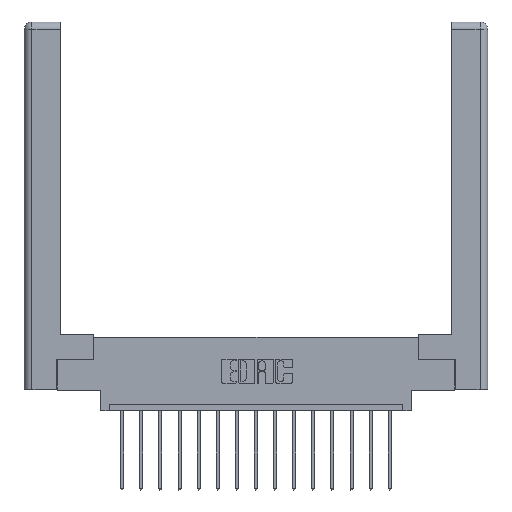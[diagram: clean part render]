
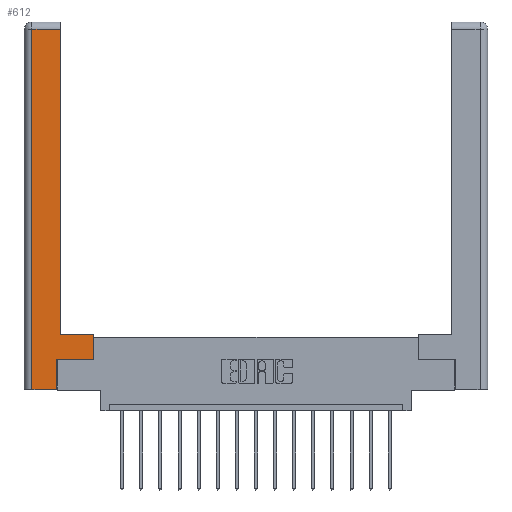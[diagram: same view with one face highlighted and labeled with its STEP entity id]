
A CAD part, top view. The second image highlights one B-rep face of the part: STEP entity #612.
In plain terms, the highlighted planar face has unit normal (0, 0, 1).
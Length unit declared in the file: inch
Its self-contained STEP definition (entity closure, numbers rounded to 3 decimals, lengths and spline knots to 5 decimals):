
#231 = VECTOR ( 'NONE', #6738, 39.37008 ) ;
#248 = CARTESIAN_POINT ( 'NONE',  ( 0.0615, 2.94, 0. ) ) ;
#262 = VECTOR ( 'NONE', #8259, 39.37008 ) ;
#455 = LINE ( 'NONE', #5295, #231 ) ;
#593 = AXIS2_PLACEMENT_3D ( 'NONE', #5013, #2111, #3486 ) ;
#612 = ADVANCED_FACE ( 'NONE', ( #8529 ), #7703, .F. ) ;
#699 = VECTOR ( 'NONE', #1119, 39.37008 ) ;
#715 = CARTESIAN_POINT ( 'NONE',  ( 0.295, 0.45, 0. ) ) ;
#750 = CARTESIAN_POINT ( 'NONE',  ( 0.565, 0.245, 0. ) ) ;
#1115 = ORIENTED_EDGE ( 'NONE', *, *, #2003, .T. ) ;
#1119 = DIRECTION ( 'NONE',  ( 0., 1., 0. ) ) ;
#1220 = EDGE_CURVE ( 'NONE', #11524, #2676, #3639, .T. ) ;
#2003 = EDGE_CURVE ( 'NONE', #2617, #9359, #12914, .T. ) ;
#2111 = DIRECTION ( 'NONE',  ( 0., 0., -1. ) ) ;
#2519 = DIRECTION ( 'NONE',  ( 0., 1., 0. ) ) ;
#2617 = VERTEX_POINT ( 'NONE', #13275 ) ;
#2668 = CARTESIAN_POINT ( 'NONE',  ( 0.565, 0.245, 0. ) ) ;
#2676 = VERTEX_POINT ( 'NONE', #3179 ) ;
#3179 = CARTESIAN_POINT ( 'NONE',  ( 0.265, 0., 0. ) ) ;
#3486 = DIRECTION ( 'NONE',  ( -1., 0., 0. ) ) ;
#3639 = LINE ( 'NONE', #13524, #10410 ) ;
#3986 = EDGE_CURVE ( 'NONE', #10735, #13105, #10806, .T. ) ;
#4422 = ORIENTED_EDGE ( 'NONE', *, *, #3986, .T. ) ;
#5013 = CARTESIAN_POINT ( 'NONE',  ( 0., 0., 0. ) ) ;
#5295 = CARTESIAN_POINT ( 'NONE',  ( 0.0615, 0., 0. ) ) ;
#5396 = ORIENTED_EDGE ( 'NONE', *, *, #7815, .T. ) ;
#5695 = ORIENTED_EDGE ( 'NONE', *, *, #13593, .T. ) ;
#5744 = LINE ( 'NONE', #2668, #262 ) ;
#5765 = ORIENTED_EDGE ( 'NONE', *, *, #1220, .T. ) ;
#6270 = VECTOR ( 'NONE', #7347, 39.37008 ) ;
#6445 = CARTESIAN_POINT ( 'NONE',  ( 0.295, 2.94, 0. ) ) ;
#6547 = EDGE_LOOP ( 'NONE', ( #1115, #6872, #5695, #5765, #7364, #7105, #4422, #5396 ) ) ;
#6738 = DIRECTION ( 'NONE',  ( 0., -1., 0. ) ) ;
#6872 = ORIENTED_EDGE ( 'NONE', *, *, #16805, .T. ) ;
#7064 = CARTESIAN_POINT ( 'NONE',  ( 0.565, 0.45, 0. ) ) ;
#7105 = ORIENTED_EDGE ( 'NONE', *, *, #12953, .T. ) ;
#7244 = VECTOR ( 'NONE', #2519, 39.37008 ) ;
#7347 = DIRECTION ( 'NONE',  ( -1., 0., 0. ) ) ;
#7364 = ORIENTED_EDGE ( 'NONE', *, *, #12517, .T. ) ;
#7703 = PLANE ( 'NONE',  #593 ) ;
#7815 = EDGE_CURVE ( 'NONE', #13105, #2617, #11560, .T. ) ;
#8259 = DIRECTION ( 'NONE',  ( 1., 0., 0. ) ) ;
#8529 = FACE_OUTER_BOUND ( 'NONE', #6547, .T. ) ;
#9359 = VERTEX_POINT ( 'NONE', #6445 ) ;
#9709 = CARTESIAN_POINT ( 'NONE',  ( 0.565, 0.45, 0. ) ) ;
#9745 = DIRECTION ( 'NONE',  ( -1., 0., 0. ) ) ;
#10025 = VECTOR ( 'NONE', #9745, 39.37008 ) ;
#10357 = CARTESIAN_POINT ( 'NONE',  ( 0.0615, 0., 0. ) ) ;
#10410 = VECTOR ( 'NONE', #15086, 39.37008 ) ;
#10695 = VERTEX_POINT ( 'NONE', #16728 ) ;
#10735 = VERTEX_POINT ( 'NONE', #750 ) ;
#10806 = LINE ( 'NONE', #9709, #12285 ) ;
#11269 = LINE ( 'NONE', #16097, #699 ) ;
#11524 = VERTEX_POINT ( 'NONE', #10357 ) ;
#11560 = LINE ( 'NONE', #715, #6270 ) ;
#12233 = VERTEX_POINT ( 'NONE', #12720 ) ;
#12285 = VECTOR ( 'NONE', #12486, 39.37008 ) ;
#12486 = DIRECTION ( 'NONE',  ( 0., 1., 0. ) ) ;
#12517 = EDGE_CURVE ( 'NONE', #2676, #12233, #11269, .T. ) ;
#12720 = CARTESIAN_POINT ( 'NONE',  ( 0.265, 0.245, 0. ) ) ;
#12914 = LINE ( 'NONE', #14315, #7244 ) ;
#12953 = EDGE_CURVE ( 'NONE', #12233, #10735, #5744, .T. ) ;
#13105 = VERTEX_POINT ( 'NONE', #7064 ) ;
#13275 = CARTESIAN_POINT ( 'NONE',  ( 0.295, 0.45, 0. ) ) ;
#13524 = CARTESIAN_POINT ( 'NONE',  ( 0.265, 0., 0. ) ) ;
#13593 = EDGE_CURVE ( 'NONE', #10695, #11524, #455, .T. ) ;
#13612 = LINE ( 'NONE', #248, #10025 ) ;
#14315 = CARTESIAN_POINT ( 'NONE',  ( 0.295, 3., 0. ) ) ;
#15086 = DIRECTION ( 'NONE',  ( 1., 0., 0. ) ) ;
#16097 = CARTESIAN_POINT ( 'NONE',  ( 0.265, 0.245, 0. ) ) ;
#16728 = CARTESIAN_POINT ( 'NONE',  ( 0.0615, 2.94, 0. ) ) ;
#16805 = EDGE_CURVE ( 'NONE', #9359, #10695, #13612, .T. ) ;
